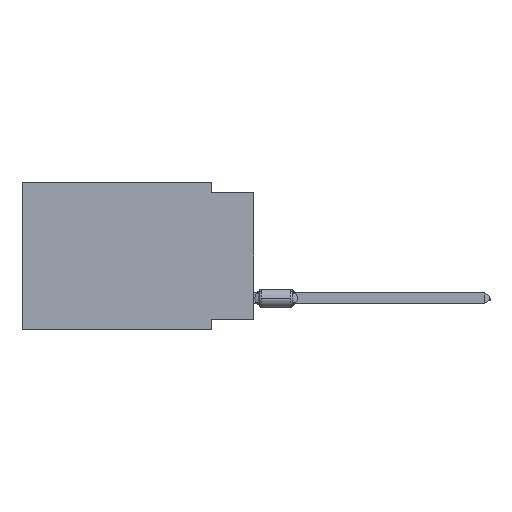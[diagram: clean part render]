
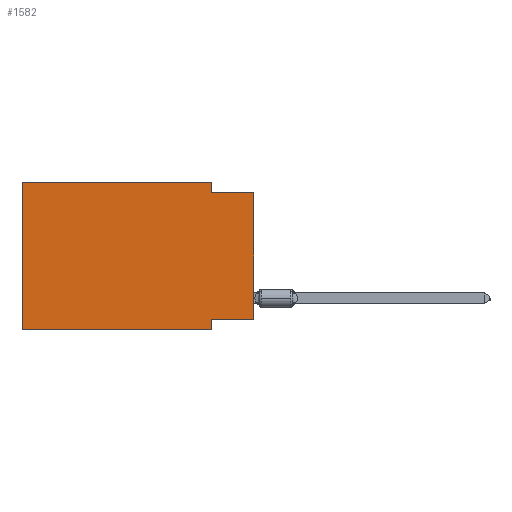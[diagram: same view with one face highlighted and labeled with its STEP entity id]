
A CAD part, left-side view. The second image highlights one B-rep face of the part: STEP entity #1582.
In plain terms, the highlighted planar face has unit normal (-1, 0, 0).
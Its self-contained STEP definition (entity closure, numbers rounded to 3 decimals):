
#909 = CARTESIAN_POINT ( 'NONE',  ( 0., 0., -8.255 ) ) ;
#1582 = ADVANCED_FACE ( 'NONE', ( #16194 ), #19763, .F. ) ;
#2535 = DIRECTION ( 'NONE',  ( 0., 0., -1. ) ) ;
#2843 = ORIENTED_EDGE ( 'NONE', *, *, #13572, .F. ) ;
#3232 = CARTESIAN_POINT ( 'NONE',  ( 0., 2.54, -8.89 ) ) ;
#3759 = CARTESIAN_POINT ( 'NONE',  ( 0., 13.97, 0. ) ) ;
#3852 = VERTEX_POINT ( 'NONE', #9881 ) ;
#6041 = CARTESIAN_POINT ( 'NONE',  ( 0., 2.54, -8.255 ) ) ;
#7199 = EDGE_CURVE ( 'NONE', #42805, #42068, #21549, .T. ) ;
#7426 = LINE ( 'NONE', #909, #38280 ) ;
#8076 = CARTESIAN_POINT ( 'NONE',  ( 0., 0., 0. ) ) ;
#9582 = CARTESIAN_POINT ( 'NONE',  ( 0., 13.97, -8.89 ) ) ;
#9736 = VECTOR ( 'NONE', #30138, 1000. ) ;
#9881 = CARTESIAN_POINT ( 'NONE',  ( 0., 2.54, -8.89 ) ) ;
#10057 = DIRECTION ( 'NONE',  ( 0., 0., 1. ) ) ;
#11082 = CARTESIAN_POINT ( 'NONE',  ( 0., 0., -0.635 ) ) ;
#11383 = LINE ( 'NONE', #11605, #22293 ) ;
#11605 = CARTESIAN_POINT ( 'NONE',  ( 0., 2.54, 0. ) ) ;
#11880 = LINE ( 'NONE', #8076, #37948 ) ;
#13349 = ORIENTED_EDGE ( 'NONE', *, *, #21561, .T. ) ;
#13572 = EDGE_CURVE ( 'NONE', #22545, #42805, #11383, .T. ) ;
#15797 = DIRECTION ( 'NONE',  ( 0., -1., 0. ) ) ;
#16137 = VERTEX_POINT ( 'NONE', #9582 ) ;
#16194 = FACE_OUTER_BOUND ( 'NONE', #19555, .T. ) ;
#16499 = EDGE_CURVE ( 'NONE', #16137, #3852, #32851, .T. ) ;
#17135 = EDGE_CURVE ( 'NONE', #37454, #41406, #7426, .T. ) ;
#17303 = VECTOR ( 'NONE', #28733, 1000. ) ;
#17380 = VECTOR ( 'NONE', #10057, 1000. ) ;
#17398 = ORIENTED_EDGE ( 'NONE', *, *, #7199, .F. ) ;
#17624 = CARTESIAN_POINT ( 'NONE',  ( 0., 13.97, 0. ) ) ;
#17752 = AXIS2_PLACEMENT_3D ( 'NONE', #29894, #43383, #2535 ) ;
#18661 = ORIENTED_EDGE ( 'NONE', *, *, #43563, .F. ) ;
#19555 = EDGE_LOOP ( 'NONE', ( #13349, #17398, #2843, #35222, #40770, #22356, #18661, #24574 ) ) ;
#19763 = PLANE ( 'NONE',  #17752 ) ;
#21549 = LINE ( 'NONE', #31639, #17303 ) ;
#21561 = EDGE_CURVE ( 'NONE', #37454, #42068, #11880, .T. ) ;
#21912 = CARTESIAN_POINT ( 'NONE',  ( 0., 2.54, -0.635 ) ) ;
#22293 = VECTOR ( 'NONE', #31362, 1000. ) ;
#22356 = ORIENTED_EDGE ( 'NONE', *, *, #16499, .T. ) ;
#22490 = CARTESIAN_POINT ( 'NONE',  ( 0., 0., -8.255 ) ) ;
#22545 = VERTEX_POINT ( 'NONE', #28481 ) ;
#23426 = VECTOR ( 'NONE', #38309, 1000. ) ;
#23807 = EDGE_CURVE ( 'NONE', #16137, #40096, #27528, .T. ) ;
#24574 = ORIENTED_EDGE ( 'NONE', *, *, #17135, .F. ) ;
#27428 = LINE ( 'NONE', #3232, #9736 ) ;
#27475 = VECTOR ( 'NONE', #15797, 1000. ) ;
#27528 = LINE ( 'NONE', #3759, #17380 ) ;
#27978 = LINE ( 'NONE', #17624, #23426 ) ;
#28481 = CARTESIAN_POINT ( 'NONE',  ( 0., 2.54, 0. ) ) ;
#28733 = DIRECTION ( 'NONE',  ( 0., -1., 0. ) ) ;
#29815 = EDGE_CURVE ( 'NONE', #40096, #22545, #27978, .T. ) ;
#29894 = CARTESIAN_POINT ( 'NONE',  ( 0., 13.97, 0. ) ) ;
#30138 = DIRECTION ( 'NONE',  ( 0., 0., -1. ) ) ;
#31362 = DIRECTION ( 'NONE',  ( 0., 0., -1. ) ) ;
#31639 = CARTESIAN_POINT ( 'NONE',  ( 0., 0., -0.635 ) ) ;
#32065 = DIRECTION ( 'NONE',  ( 0., 0., 1. ) ) ;
#32851 = LINE ( 'NONE', #42968, #27475 ) ;
#35222 = ORIENTED_EDGE ( 'NONE', *, *, #29815, .F. ) ;
#37454 = VERTEX_POINT ( 'NONE', #22490 ) ;
#37948 = VECTOR ( 'NONE', #32065, 1000. ) ;
#38280 = VECTOR ( 'NONE', #41982, 1000. ) ;
#38309 = DIRECTION ( 'NONE',  ( 0., -1., 0. ) ) ;
#40096 = VERTEX_POINT ( 'NONE', #40974 ) ;
#40770 = ORIENTED_EDGE ( 'NONE', *, *, #23807, .F. ) ;
#40974 = CARTESIAN_POINT ( 'NONE',  ( 0., 13.97, 0. ) ) ;
#41406 = VERTEX_POINT ( 'NONE', #6041 ) ;
#41982 = DIRECTION ( 'NONE',  ( 0., 1., 0. ) ) ;
#42068 = VERTEX_POINT ( 'NONE', #11082 ) ;
#42805 = VERTEX_POINT ( 'NONE', #21912 ) ;
#42968 = CARTESIAN_POINT ( 'NONE',  ( 0., 13.97, -8.89 ) ) ;
#43383 = DIRECTION ( 'NONE',  ( 1., 0., 0. ) ) ;
#43563 = EDGE_CURVE ( 'NONE', #41406, #3852, #27428, .T. ) ;
